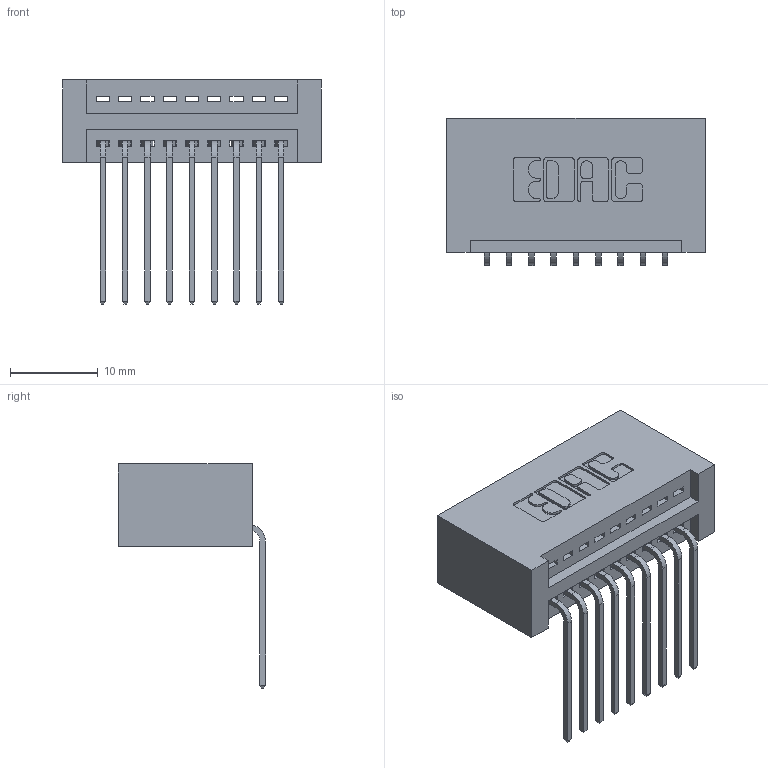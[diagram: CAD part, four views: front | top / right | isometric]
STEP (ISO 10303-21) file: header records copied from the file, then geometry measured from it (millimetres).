
FILE_DESCRIPTION (( 'STEP AP203' ), '1' );
FILE_NAME ('345-009-559-101.STEP', '2019-10-03T20:55:49', ( '' ), ( '' ), 'SwSTEP 2.0', 'SolidWorks 2016', '' );
FILE_SCHEMA (( 'CONFIG_CONTROL_DESIGN' ));
Length unit declared in the file: inch
Products named in the file (3): 345-292-001_558 559 Tail - 1; 345-009-559-101; 345 Part_No Mounting Lugs
Assembly tree (10 placements, depth 2):
  345-009-559-101
    345 Part_No Mounting Lugs
    345-292-001_558 559 Tail - 1  x9
Bounding box: 29.46 x 16.75 x 25.53 mm (x, y, z)
Volume: 3142.5 mm3; surface area: 4094 mm2
Topology: 10 solids, 10 shells, 658 faces, 1955 edges, 1290 vertices
Faces by surface type: plane 454, cylinder 204
Entity records: 11023 total; most frequent: CARTESIAN_POINT 1919, ORIENTED_EDGE 1862, DIRECTION 1717, EDGE_CURVE 931, VECTOR 771, LINE 771, VERTEX_POINT 618, AXIS2_PLACEMENT_3D 473
